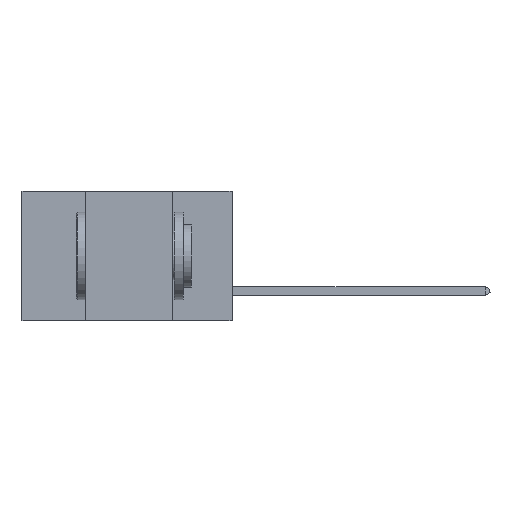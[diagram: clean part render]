
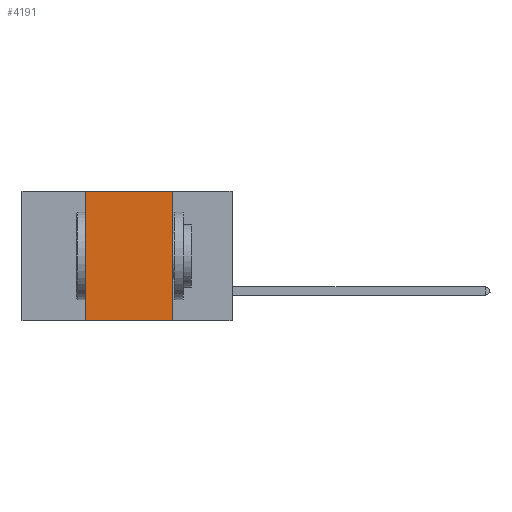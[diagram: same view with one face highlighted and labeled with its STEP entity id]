
A CAD part, left-side view. The second image highlights one B-rep face of the part: STEP entity #4191.
In plain terms, the highlighted planar face has unit normal (-1, 0, 0).
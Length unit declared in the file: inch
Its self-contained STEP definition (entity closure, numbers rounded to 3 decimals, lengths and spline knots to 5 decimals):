
#843 = DIRECTION ( 'NONE',  ( 1., 0., 0. ) ) ;
#921 = PLANE ( 'NONE',  #1411 ) ;
#986 = DIRECTION ( 'NONE',  ( 0., -1., 0. ) ) ;
#1111 = CARTESIAN_POINT ( 'NONE',  ( 0., 0.6, -0.37 ) ) ;
#1266 = CARTESIAN_POINT ( 'NONE',  ( 0., 0.17, -0.37 ) ) ;
#1411 = AXIS2_PLACEMENT_3D ( 'NONE', #6484, #843, #8358 ) ;
#1536 = VERTEX_POINT ( 'NONE', #9203 ) ;
#2299 = DIRECTION ( 'NONE',  ( 0., 0., -1. ) ) ;
#2641 = VECTOR ( 'NONE', #7468, 39.37008 ) ;
#3329 = VERTEX_POINT ( 'NONE', #3811 ) ;
#3811 = CARTESIAN_POINT ( 'NONE',  ( 0., 0.42, -0.37 ) ) ;
#4191 = ADVANCED_FACE ( 'NONE', ( #9873 ), #921, .F. ) ;
#4226 = EDGE_CURVE ( 'NONE', #3329, #8470, #8171, .T. ) ;
#4444 = LINE ( 'NONE', #9564, #11532 ) ;
#4471 = EDGE_LOOP ( 'NONE', ( #6374, #7132, #8132, #6864 ) ) ;
#5672 = CARTESIAN_POINT ( 'NONE',  ( 0., 0.42, 0. ) ) ;
#5766 = EDGE_CURVE ( 'NONE', #3329, #7890, #7870, .T. ) ;
#5781 = VECTOR ( 'NONE', #10532, 39.37008 ) ;
#6374 = ORIENTED_EDGE ( 'NONE', *, *, #7190, .F. ) ;
#6484 = CARTESIAN_POINT ( 'NONE',  ( 0., 0.6, 0. ) ) ;
#6645 = LINE ( 'NONE', #11163, #2641 ) ;
#6864 = ORIENTED_EDGE ( 'NONE', *, *, #5766, .T. ) ;
#7132 = ORIENTED_EDGE ( 'NONE', *, *, #10250, .F. ) ;
#7154 = VECTOR ( 'NONE', #986, 39.37008 ) ;
#7190 = EDGE_CURVE ( 'NONE', #1536, #7890, #4444, .T. ) ;
#7468 = DIRECTION ( 'NONE',  ( 0., -1., 0. ) ) ;
#7822 = CARTESIAN_POINT ( 'NONE',  ( 0., 0.42, 0. ) ) ;
#7870 = LINE ( 'NONE', #1111, #7154 ) ;
#7890 = VERTEX_POINT ( 'NONE', #1266 ) ;
#8132 = ORIENTED_EDGE ( 'NONE', *, *, #4226, .F. ) ;
#8171 = LINE ( 'NONE', #7822, #5781 ) ;
#8358 = DIRECTION ( 'NONE',  ( 0., 0., -1. ) ) ;
#8470 = VERTEX_POINT ( 'NONE', #5672 ) ;
#9203 = CARTESIAN_POINT ( 'NONE',  ( 0., 0.17, 0. ) ) ;
#9564 = CARTESIAN_POINT ( 'NONE',  ( 0., 0.17, 0. ) ) ;
#9873 = FACE_OUTER_BOUND ( 'NONE', #4471, .T. ) ;
#10250 = EDGE_CURVE ( 'NONE', #8470, #1536, #6645, .T. ) ;
#10532 = DIRECTION ( 'NONE',  ( 0., 0., 1. ) ) ;
#11163 = CARTESIAN_POINT ( 'NONE',  ( 0., 0.6, 0. ) ) ;
#11532 = VECTOR ( 'NONE', #2299, 39.37008 ) ;
